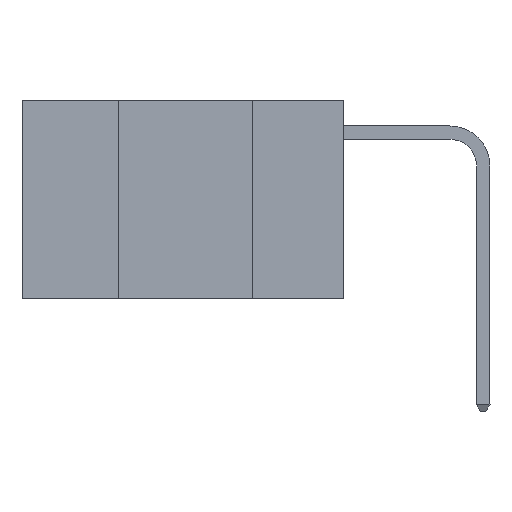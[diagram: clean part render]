
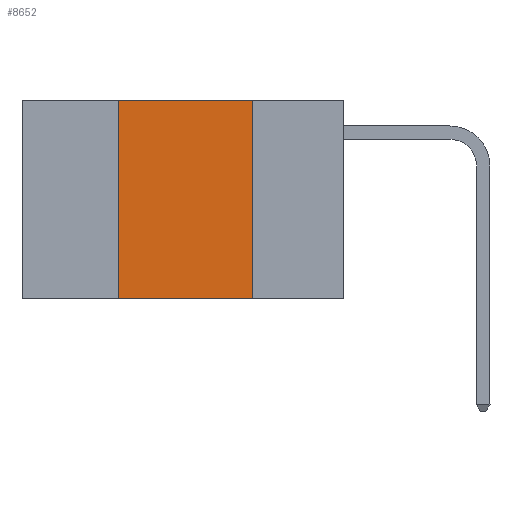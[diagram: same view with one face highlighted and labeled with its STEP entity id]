
A CAD part, left-side view. The second image highlights one B-rep face of the part: STEP entity #8652.
In plain terms, the highlighted planar face has unit normal (-1, 0, 0).
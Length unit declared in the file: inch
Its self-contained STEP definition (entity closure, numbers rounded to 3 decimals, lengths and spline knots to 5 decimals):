
#301 = LINE ( 'NONE', #3910, #3884 ) ;
#431 = VECTOR ( 'NONE', #3704, 39.37008 ) ;
#698 = EDGE_CURVE ( 'NONE', #5195, #9123, #6657, .T. ) ;
#1196 = ORIENTED_EDGE ( 'NONE', *, *, #2039, .F. ) ;
#1230 = CARTESIAN_POINT ( 'NONE',  ( 0., 0.42, 0. ) ) ;
#1235 = DIRECTION ( 'NONE',  ( 0., 0., -1. ) ) ;
#1652 = ORIENTED_EDGE ( 'NONE', *, *, #11154, .T. ) ;
#1966 = CARTESIAN_POINT ( 'NONE',  ( 0., 0.17, 0. ) ) ;
#2039 = EDGE_CURVE ( 'NONE', #10850, #4369, #4846, .T. ) ;
#2078 = LINE ( 'NONE', #2986, #7466 ) ;
#2145 = CARTESIAN_POINT ( 'NONE',  ( 0., 0.6, 0. ) ) ;
#2200 = DIRECTION ( 'NONE',  ( 0., -1., 0. ) ) ;
#2716 = CARTESIAN_POINT ( 'NONE',  ( 0., 0.42, -0.37 ) ) ;
#2986 = CARTESIAN_POINT ( 'NONE',  ( 0., 0.6, 0. ) ) ;
#3704 = DIRECTION ( 'NONE',  ( 0., 0., 1. ) ) ;
#3884 = VECTOR ( 'NONE', #8506, 39.37008 ) ;
#3910 = CARTESIAN_POINT ( 'NONE',  ( 0., 0.6, -0.37 ) ) ;
#4002 = PLANE ( 'NONE',  #9084 ) ;
#4369 = VERTEX_POINT ( 'NONE', #11811 ) ;
#4480 = EDGE_CURVE ( 'NONE', #9123, #10850, #2078, .T. ) ;
#4846 = LINE ( 'NONE', #1966, #5418 ) ;
#5195 = VERTEX_POINT ( 'NONE', #2716 ) ;
#5418 = VECTOR ( 'NONE', #1235, 39.37008 ) ;
#5770 = EDGE_LOOP ( 'NONE', ( #1196, #6963, #11637, #1652 ) ) ;
#6657 = LINE ( 'NONE', #11257, #431 ) ;
#6725 = DIRECTION ( 'NONE',  ( 1., 0., 0. ) ) ;
#6963 = ORIENTED_EDGE ( 'NONE', *, *, #4480, .F. ) ;
#7466 = VECTOR ( 'NONE', #2200, 39.37008 ) ;
#8506 = DIRECTION ( 'NONE',  ( 0., -1., 0. ) ) ;
#8652 = ADVANCED_FACE ( 'NONE', ( #9522 ), #4002, .F. ) ;
#9084 = AXIS2_PLACEMENT_3D ( 'NONE', #2145, #6725, #9401 ) ;
#9123 = VERTEX_POINT ( 'NONE', #1230 ) ;
#9401 = DIRECTION ( 'NONE',  ( 0., 0., -1. ) ) ;
#9522 = FACE_OUTER_BOUND ( 'NONE', #5770, .T. ) ;
#10850 = VERTEX_POINT ( 'NONE', #11716 ) ;
#11154 = EDGE_CURVE ( 'NONE', #5195, #4369, #301, .T. ) ;
#11257 = CARTESIAN_POINT ( 'NONE',  ( 0., 0.42, 0. ) ) ;
#11637 = ORIENTED_EDGE ( 'NONE', *, *, #698, .F. ) ;
#11716 = CARTESIAN_POINT ( 'NONE',  ( 0., 0.17, 0. ) ) ;
#11811 = CARTESIAN_POINT ( 'NONE',  ( 0., 0.17, -0.37 ) ) ;
